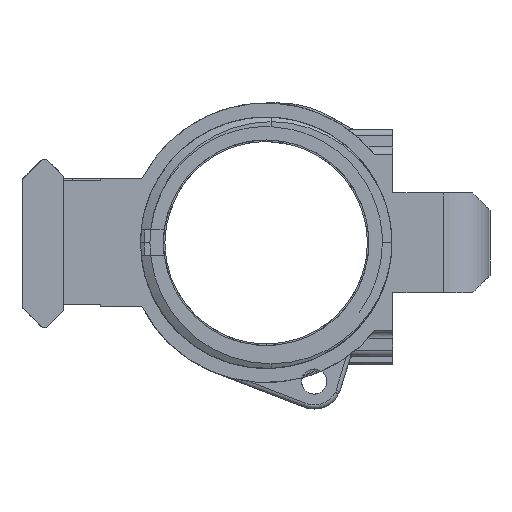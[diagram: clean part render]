
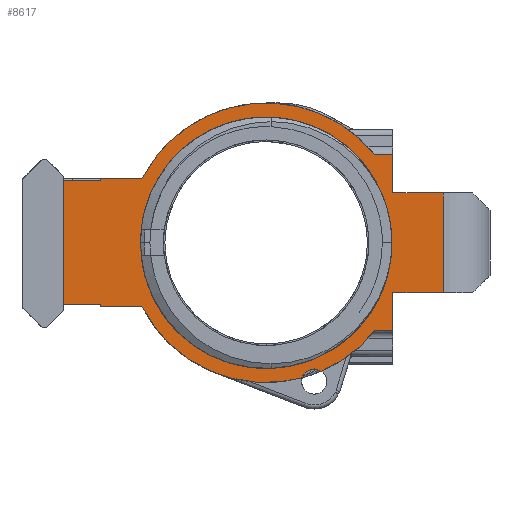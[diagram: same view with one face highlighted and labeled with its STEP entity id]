
A CAD part, left-side view. The second image highlights one B-rep face of the part: STEP entity #8617.
In plain terms, the highlighted planar face has unit normal (-1, 0, 0).
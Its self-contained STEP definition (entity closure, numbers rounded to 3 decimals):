
#27=FACE_BOUND('',#1433,.T.);
#562=PLANE('',#9293);
#971=FACE_OUTER_BOUND('',#1432,.T.);
#1432=EDGE_LOOP('',(#7482,#7483,#7484,#7485,#7486,#7487,#7488,#7489,#7490,
#7491,#7492,#7493,#7494,#7495,#7496,#7497,#7498,#7499,#7500,#7501,#7502,
#7503,#7504));
#1433=EDGE_LOOP('',(#7505));
#1999=LINE('',#15530,#2812);
#2002=LINE('',#15537,#2815);
#2003=LINE('',#15541,#2816);
#2004=LINE('',#15546,#2817);
#2008=LINE('',#15553,#2821);
#2014=LINE('',#15572,#2827);
#2019=LINE('',#15585,#2832);
#2020=LINE('',#15588,#2833);
#2024=LINE('',#15600,#2837);
#2057=LINE('',#15935,#2870);
#2059=LINE('',#15939,#2872);
#2092=LINE('',#16025,#2905);
#2171=LINE('',#16595,#2984);
#2172=LINE('',#16596,#2985);
#2199=LINE('',#17338,#3012);
#2200=LINE('',#17340,#3013);
#2201=LINE('',#17344,#3014);
#2202=LINE('',#17345,#3015);
#2812=VECTOR('',#10681,10.);
#2815=VECTOR('',#10688,10.);
#2816=VECTOR('',#10693,12.548);
#2817=VECTOR('',#10700,10.);
#2821=VECTOR('',#10706,10.);
#2827=VECTOR('',#10724,10.);
#2832=VECTOR('',#10735,10.);
#2833=VECTOR('',#10738,10.);
#2837=VECTOR('',#10748,10.);
#2870=VECTOR('',#10831,10.);
#2872=VECTOR('',#10835,10.);
#2905=VECTOR('',#10916,10.);
#2984=VECTOR('',#11161,10.);
#2985=VECTOR('',#11162,10.);
#3012=VECTOR('',#11253,10.);
#3013=VECTOR('',#11256,10.);
#3014=VECTOR('',#11259,10.);
#3015=VECTOR('',#11260,10.);
#3270=CIRCLE('',#9105,14.891);
#3275=CIRCLE('',#9116,17.621);
#3276=CIRCLE('',#9118,1.588);
#3277=CIRCLE('',#9119,1.588);
#3299=CIRCLE('',#9179,17.621);
#3347=CIRCLE('',#9294,17.621);
#3882=VERTEX_POINT('',#15509);
#3886=VERTEX_POINT('',#15527);
#3887=VERTEX_POINT('',#15529);
#3888=VERTEX_POINT('',#15534);
#3889=VERTEX_POINT('',#15536);
#3890=VERTEX_POINT('',#15540);
#3891=VERTEX_POINT('',#15545);
#3892=VERTEX_POINT('',#15549);
#3893=VERTEX_POINT('',#15551);
#3894=VERTEX_POINT('',#15555);
#3895=VERTEX_POINT('',#15559);
#3896=VERTEX_POINT('',#15562);
#3899=VERTEX_POINT('',#15569);
#3900=VERTEX_POINT('',#15571);
#3901=VERTEX_POINT('',#15575);
#3906=VERTEX_POINT('',#15587);
#3911=VERTEX_POINT('',#15599);
#3946=VERTEX_POINT('',#15933);
#3947=VERTEX_POINT('',#15937);
#3976=VERTEX_POINT('',#16023);
#4068=VERTEX_POINT('',#16593);
#4109=VERTEX_POINT('',#17336);
#4110=VERTEX_POINT('',#17341);
#4111=VERTEX_POINT('',#17343);
#4971=EDGE_CURVE('',#3882,#3882,#3270,.T.);
#4975=EDGE_CURVE('',#3887,#3886,#1999,.T.);
#4979=EDGE_CURVE('',#3889,#3888,#2002,.F.);
#4981=EDGE_CURVE('',#3890,#3889,#2003,.T.);
#4984=EDGE_CURVE('',#3891,#3890,#2004,.F.);
#4988=EDGE_CURVE('',#3892,#3893,#2008,.F.);
#4989=EDGE_CURVE('',#3892,#3894,#3275,.T.);
#4991=EDGE_CURVE('',#3894,#3895,#3276,.F.);
#4993=EDGE_CURVE('',#3895,#3896,#3277,.F.);
#4997=EDGE_CURVE('',#3900,#3899,#2014,.T.);
#5004=EDGE_CURVE('',#3900,#3901,#2019,.T.);
#5005=EDGE_CURVE('',#3906,#3901,#2020,.T.);
#5011=EDGE_CURVE('',#3911,#3887,#2024,.T.);
#5063=EDGE_CURVE('',#3946,#3886,#2057,.T.);
#5065=EDGE_CURVE('',#3906,#3947,#2059,.T.);
#5108=EDGE_CURVE('',#3976,#3899,#2092,.T.);
#5109=EDGE_CURVE('',#3896,#3976,#3299,.T.);
#5242=EDGE_CURVE('',#4068,#3888,#2171,.T.);
#5243=EDGE_CURVE('',#3891,#3893,#2172,.T.);
#5306=EDGE_CURVE('',#4068,#4109,#2199,.F.);
#5307=EDGE_CURVE('',#3946,#3947,#2200,.T.);
#5308=EDGE_CURVE('',#4110,#4109,#3347,.T.);
#5309=EDGE_CURVE('',#4110,#4111,#2201,.F.);
#5310=EDGE_CURVE('',#4111,#3911,#2202,.T.);
#7482=ORIENTED_EDGE('',*,*,#5307,.T.);
#7483=ORIENTED_EDGE('',*,*,#5065,.F.);
#7484=ORIENTED_EDGE('',*,*,#5005,.T.);
#7485=ORIENTED_EDGE('',*,*,#5004,.F.);
#7486=ORIENTED_EDGE('',*,*,#4997,.T.);
#7487=ORIENTED_EDGE('',*,*,#5108,.F.);
#7488=ORIENTED_EDGE('',*,*,#5109,.F.);
#7489=ORIENTED_EDGE('',*,*,#4993,.F.);
#7490=ORIENTED_EDGE('',*,*,#4991,.F.);
#7491=ORIENTED_EDGE('',*,*,#4989,.F.);
#7492=ORIENTED_EDGE('',*,*,#4988,.T.);
#7493=ORIENTED_EDGE('',*,*,#5243,.F.);
#7494=ORIENTED_EDGE('',*,*,#4984,.T.);
#7495=ORIENTED_EDGE('',*,*,#4981,.T.);
#7496=ORIENTED_EDGE('',*,*,#4979,.T.);
#7497=ORIENTED_EDGE('',*,*,#5242,.F.);
#7498=ORIENTED_EDGE('',*,*,#5306,.T.);
#7499=ORIENTED_EDGE('',*,*,#5308,.F.);
#7500=ORIENTED_EDGE('',*,*,#5309,.T.);
#7501=ORIENTED_EDGE('',*,*,#5310,.T.);
#7502=ORIENTED_EDGE('',*,*,#5011,.T.);
#7503=ORIENTED_EDGE('',*,*,#4975,.T.);
#7504=ORIENTED_EDGE('',*,*,#5063,.F.);
#7505=ORIENTED_EDGE('',*,*,#4971,.T.);
#8617=ADVANCED_FACE('',(#971,#27),#562,.F.);
#9105=AXIS2_PLACEMENT_3D('',#15511,#10675,#10676);
#9116=AXIS2_PLACEMENT_3D('',#15556,#10709,#10710);
#9118=AXIS2_PLACEMENT_3D('',#15560,#10714,#10715);
#9119=AXIS2_PLACEMENT_3D('',#15563,#10717,#10718);
#9179=AXIS2_PLACEMENT_3D('',#16027,#10919,#10920);
#9293=AXIS2_PLACEMENT_3D('',#17339,#11254,#11255);
#9294=AXIS2_PLACEMENT_3D('',#17342,#11257,#11258);
#10675=DIRECTION('center_axis',(1.,0.,0.));
#10676=DIRECTION('ref_axis',(0.,0.,1.));
#10681=DIRECTION('',(0.,0.,1.));
#10688=DIRECTION('',(0.,-1.,0.));
#10693=DIRECTION('',(0.,0.,1.));
#10700=DIRECTION('',(0.,1.,0.));
#10706=DIRECTION('',(0.,1.,0.));
#10709=DIRECTION('center_axis',(1.,0.,0.));
#10710=DIRECTION('ref_axis',(0.,0.,-1.));
#10714=DIRECTION('center_axis',(1.,0.,0.));
#10715=DIRECTION('ref_axis',(0.,0.,-1.));
#10717=DIRECTION('center_axis',(1.,0.,0.));
#10718=DIRECTION('ref_axis',(0.,0.,-1.));
#10724=DIRECTION('',(0.,0.,-1.));
#10735=DIRECTION('',(0.,1.,0.));
#10738=DIRECTION('',(0.,0.,1.));
#10748=DIRECTION('',(0.,1.,0.));
#10831=DIRECTION('',(0.,-1.,0.));
#10835=DIRECTION('',(0.,1.,0.));
#10916=DIRECTION('',(0.,1.,0.));
#10919=DIRECTION('center_axis',(1.,0.,0.));
#10920=DIRECTION('ref_axis',(0.,0.,-1.));
#11161=DIRECTION('',(0.,0.,-1.));
#11162=DIRECTION('',(0.,0.,-1.));
#11253=DIRECTION('',(0.,-1.,0.));
#11254=DIRECTION('center_axis',(1.,0.,0.));
#11255=DIRECTION('ref_axis',(0.,0.,-1.));
#11256=DIRECTION('',(0.,0.,-1.));
#11257=DIRECTION('center_axis',(1.,0.,0.));
#11258=DIRECTION('ref_axis',(0.,0.,1.));
#11259=DIRECTION('',(0.,-1.,0.));
#11260=DIRECTION('',(0.,0.,-1.));
#15509=CARTESIAN_POINT('',(393.794,184.018,-1.102));
#15511=CARTESIAN_POINT('Origin',(393.794,184.018,13.789));
#15527=CARTESIAN_POINT('',(393.794,209.571,21.879));
#15529=CARTESIAN_POINT('',(393.794,209.571,21.625));
#15530=CARTESIAN_POINT('',(393.794,209.571,9.995));
#15534=CARTESIAN_POINT('',(393.794,168.042,20.063));
#15536=CARTESIAN_POINT('',(393.794,161.692,20.063));
#15537=CARTESIAN_POINT('',(393.794,164.867,20.063));
#15540=CARTESIAN_POINT('',(393.794,161.692,7.515));
#15541=CARTESIAN_POINT('',(393.794,161.692,7.515));
#15545=CARTESIAN_POINT('',(393.794,168.042,7.515));
#15546=CARTESIAN_POINT('',(393.794,159.838,7.515));
#15549=CARTESIAN_POINT('',(393.794,170.343,2.676));
#15551=CARTESIAN_POINT('',(393.794,168.042,2.676));
#15553=CARTESIAN_POINT('',(393.794,164.867,2.676));
#15555=CARTESIAN_POINT('',(393.794,177.06,-2.4));
#15556=CARTESIAN_POINT('Origin',(393.794,184.018,13.789));
#15559=CARTESIAN_POINT('',(393.794,177.963,-2.119));
#15560=CARTESIAN_POINT('Origin',(393.794,177.963,-3.706));
#15562=CARTESIAN_POINT('',(393.794,179.48,-3.238));
#15563=CARTESIAN_POINT('Origin',(393.794,177.963,-3.706));
#15569=CARTESIAN_POINT('',(393.794,204.872,5.699));
#15571=CARTESIAN_POINT('',(393.794,204.872,5.953));
#15572=CARTESIAN_POINT('',(393.794,204.872,2.159));
#15575=CARTESIAN_POINT('',(393.794,209.571,5.953));
#15585=CARTESIAN_POINT('',(393.794,183.282,5.953));
#15587=CARTESIAN_POINT('',(393.794,209.571,5.699));
#15588=CARTESIAN_POINT('',(393.794,209.571,1.848));
#15599=CARTESIAN_POINT('',(393.794,204.872,21.625));
#15600=CARTESIAN_POINT('',(393.794,183.282,21.625));
#15933=CARTESIAN_POINT('',(393.794,209.594,21.879));
#15935=CARTESIAN_POINT('',(393.794,180.139,21.879));
#15937=CARTESIAN_POINT('',(393.794,209.594,5.699));
#15939=CARTESIAN_POINT('',(393.794,179.808,5.699));
#16023=CARTESIAN_POINT('',(393.794,199.673,5.699));
#16025=CARTESIAN_POINT('',(393.794,180.139,5.699));
#16027=CARTESIAN_POINT('Origin',(393.794,184.018,13.789));
#16593=CARTESIAN_POINT('',(393.794,168.042,24.901));
#16595=CARTESIAN_POINT('',(393.794,168.042,-1.067));
#16596=CARTESIAN_POINT('',(393.794,168.042,-1.067));
#17336=CARTESIAN_POINT('',(393.794,170.343,24.901));
#17338=CARTESIAN_POINT('',(393.794,167.276,24.901));
#17339=CARTESIAN_POINT('Origin',(393.794,161.692,-1.635));
#17340=CARTESIAN_POINT('',(393.794,209.594,1.816));
#17341=CARTESIAN_POINT('',(393.794,199.673,21.879));
#17342=CARTESIAN_POINT('Origin',(393.794,184.018,13.789));
#17343=CARTESIAN_POINT('',(393.794,204.872,21.879));
#17344=CARTESIAN_POINT('',(393.794,183.282,21.879));
#17345=CARTESIAN_POINT('',(393.794,204.872,10.122));
